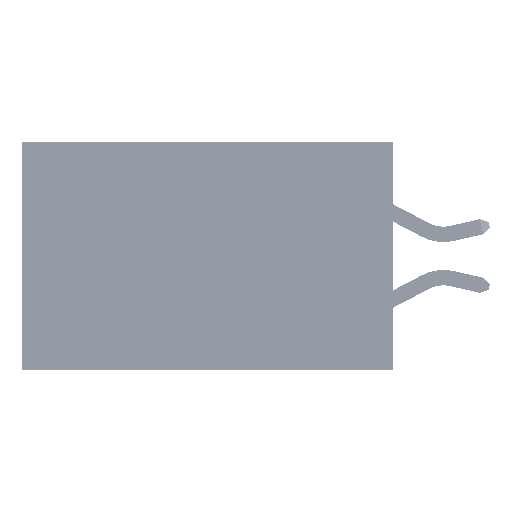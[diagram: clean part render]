
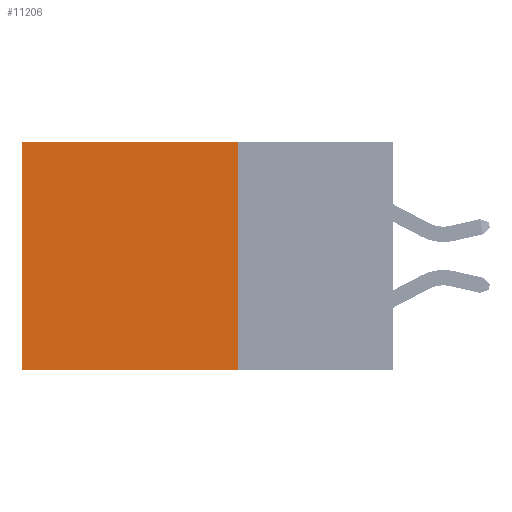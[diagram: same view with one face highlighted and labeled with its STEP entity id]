
A CAD part, left-side view. The second image highlights one B-rep face of the part: STEP entity #11206.
In plain terms, the highlighted planar face has unit normal (-1, 0, 0).
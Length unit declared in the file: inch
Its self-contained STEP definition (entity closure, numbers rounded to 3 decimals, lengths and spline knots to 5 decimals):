
#129 = ORIENTED_EDGE ( 'NONE', *, *, #10804, .F. ) ;
#2690 = VERTEX_POINT ( 'NONE', #31000 ) ;
#2852 = CARTESIAN_POINT ( 'NONE',  ( 0.2875, 0.6, 0. ) ) ;
#3066 = ORIENTED_EDGE ( 'NONE', *, *, #3852, .T. ) ;
#3539 = DIRECTION ( 'NONE',  ( 0., 1., 0. ) ) ;
#3830 = DIRECTION ( 'NONE',  ( 0., 0., -1. ) ) ;
#3852 = EDGE_CURVE ( 'NONE', #15274, #2690, #21752, .T. ) ;
#7736 = CARTESIAN_POINT ( 'NONE',  ( 0.2875, 0.25, -0.37 ) ) ;
#10648 = VECTOR ( 'NONE', #32325, 39.37008 ) ;
#10804 = EDGE_CURVE ( 'NONE', #25888, #2690, #45462, .T. ) ;
#11206 = ADVANCED_FACE ( 'NONE', ( #38266 ), #30862, .F. ) ;
#11526 = EDGE_CURVE ( 'NONE', #43020, #25888, #13378, .T. ) ;
#13112 = CARTESIAN_POINT ( 'NONE',  ( 0.2875, 0.25, 0. ) ) ;
#13309 = EDGE_LOOP ( 'NONE', ( #3066, #129, #17768, #52705 ) ) ;
#13378 = LINE ( 'NONE', #33003, #23170 ) ;
#14257 = CARTESIAN_POINT ( 'NONE',  ( 0.2875, 0.25, 0. ) ) ;
#15274 = VERTEX_POINT ( 'NONE', #2852 ) ;
#15547 = CARTESIAN_POINT ( 'NONE',  ( 0.2875, 0.6, 0. ) ) ;
#17768 = ORIENTED_EDGE ( 'NONE', *, *, #11526, .F. ) ;
#20442 = VECTOR ( 'NONE', #42227, 39.37008 ) ;
#21752 = LINE ( 'NONE', #15547, #10648 ) ;
#23170 = VECTOR ( 'NONE', #3830, 39.37008 ) ;
#23354 = VECTOR ( 'NONE', #3539, 39.37008 ) ;
#25888 = VERTEX_POINT ( 'NONE', #40785 ) ;
#26861 = DIRECTION ( 'NONE',  ( 0., 0., -1. ) ) ;
#30862 = PLANE ( 'NONE',  #45491 ) ;
#30936 = EDGE_CURVE ( 'NONE', #43020, #15274, #31521, .T. ) ;
#31000 = CARTESIAN_POINT ( 'NONE',  ( 0.2875, 0.6, -0.37 ) ) ;
#31521 = LINE ( 'NONE', #13112, #20442 ) ;
#32325 = DIRECTION ( 'NONE',  ( 0., 0., -1. ) ) ;
#33003 = CARTESIAN_POINT ( 'NONE',  ( 0.2875, 0.25, 0. ) ) ;
#38266 = FACE_OUTER_BOUND ( 'NONE', #13309, .T. ) ;
#39332 = CARTESIAN_POINT ( 'NONE',  ( 0.2875, 0.25, 0. ) ) ;
#40785 = CARTESIAN_POINT ( 'NONE',  ( 0.2875, 0.25, -0.37 ) ) ;
#42227 = DIRECTION ( 'NONE',  ( 0., 1., 0. ) ) ;
#43020 = VERTEX_POINT ( 'NONE', #39332 ) ;
#45462 = LINE ( 'NONE', #7736, #23354 ) ;
#45491 = AXIS2_PLACEMENT_3D ( 'NONE', #14257, #51711, #26861 ) ;
#51711 = DIRECTION ( 'NONE',  ( 1., 0., 0. ) ) ;
#52705 = ORIENTED_EDGE ( 'NONE', *, *, #30936, .T. ) ;
